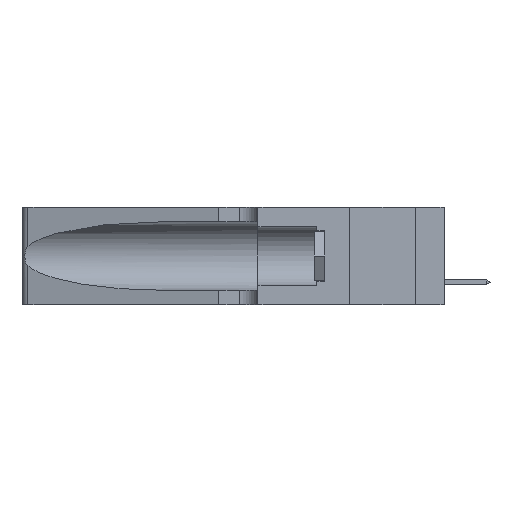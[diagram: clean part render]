
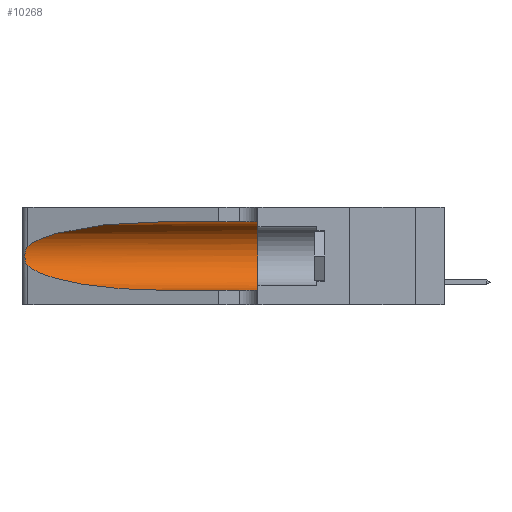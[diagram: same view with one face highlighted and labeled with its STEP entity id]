
A CAD part, left-side view. The second image highlights one B-rep face of the part: STEP entity #10268.
In plain terms, the highlighted cylindrical face has radius 3.308 mm (diameter 6.617 mm), a partial arc.
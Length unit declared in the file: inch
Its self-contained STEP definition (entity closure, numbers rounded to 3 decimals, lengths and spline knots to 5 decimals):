
#1275 = CARTESIAN_POINT ( 'NONE',  ( 0.1305, 0.72297, 0.05475 ) ) ;
#1622 = ORIENTED_EDGE ( 'NONE', *, *, #4920, .T. ) ;
#1725 = CARTESIAN_POINT ( 'NONE',  ( 0.26017, 1.23833, 0.17102 ) ) ;
#1914 = DIRECTION ( 'NONE',  ( 0., 0., -1. ) ) ;
#2087 = LINE ( 'NONE', #11786, #18415 ) ;
#2532 = CARTESIAN_POINT ( 'NONE',  ( 0.25787, 1.23484, 0.2124 ) ) ;
#2610 = CARTESIAN_POINT ( 'NONE',  ( 0.26075, 1.23896, 0.19203 ) ) ;
#3194 = CARTESIAN_POINT ( 'NONE',  ( 0.25487, 1.22718, 0.14631 ) ) ;
#3207 = ORIENTED_EDGE ( 'NONE', *, *, #10612, .T. ) ;
#3215 = CARTESIAN_POINT ( 'NONE',  ( 0.25487, 1.22718, 0.14631 ) ) ;
#3239 = CARTESIAN_POINT ( 'NONE',  ( 0.1305, 0.72297, 0.31525 ) ) ;
#3676 = CARTESIAN_POINT ( 'NONE',  ( 0.2373, 1.15595, 0.28018 ) ) ;
#4524 = EDGE_LOOP ( 'NONE', ( #3207, #1622, #17276, #13092, #5275, #13192 ) ) ;
#4920 = EDGE_CURVE ( 'NONE', #6369, #17514, #17441, .T. ) ;
#5008 = CARTESIAN_POINT ( 'NONE',  ( 0.1305, 1.61858, 0.185 ) ) ;
#5275 = ORIENTED_EDGE ( 'NONE', *, *, #12009, .F. ) ;
#5328 = DIRECTION ( 'NONE',  ( 0., -1., 0. ) ) ;
#5512 = VERTEX_POINT ( 'NONE', #19011 ) ;
#5813 = VERTEX_POINT ( 'NONE', #1275 ) ;
#5900 = FACE_OUTER_BOUND ( 'NONE', #4524, .T. ) ;
#5955 = EDGE_CURVE ( 'NONE', #17514, #5813, #17702, .T. ) ;
#6369 = VERTEX_POINT ( 'NONE', #16357 ) ;
#7639 = CYLINDRICAL_SURFACE ( 'NONE', #16530, 0.13025 ) ;
#7770 = EDGE_CURVE ( 'NONE', #17005, #5512, #19348, .T. ) ;
#9544 = CARTESIAN_POINT ( 'NONE',  ( 0.25856, 1.23593, 0.16098 ) ) ;
#9604 = CARTESIAN_POINT ( 'NONE',  ( 0.25789, 1.23486, 0.15765 ) ) ;
#9733 = CARTESIAN_POINT ( 'NONE',  ( 0.25487, 1.22718, 0.22369 ) ) ;
#9821 = CARTESIAN_POINT ( 'NONE',  ( 0.18966, 0.96281, 0.05475 ) ) ;
#9995 = VECTOR ( 'NONE', #5328, 39.37008 ) ;
#10268 = ADVANCED_FACE ( 'NONE', ( #5900 ), #7639, .F. ) ;
#10290 = CARTESIAN_POINT ( 'NONE',  ( 0.25487, 1.22718, 0.22369 ) ) ;
#10612 = EDGE_CURVE ( 'NONE', #17005, #6369, #12275, .T. ) ;
#11355 = CARTESIAN_POINT ( 'NONE',  ( 0.18966, 0.96281, 0.31525 ) ) ;
#11786 = CARTESIAN_POINT ( 'NONE',  ( 0.1305, 1.61858, 0.05475 ) ) ;
#12009 = EDGE_CURVE ( 'NONE', #5512, #19830, #14954, .T. ) ;
#12275 =( BOUNDED_CURVE ( )  B_SPLINE_CURVE ( 3, ( #19216, #11355, #3676, #9733 ),
 .UNSPECIFIED., .F., .F. ) 
 B_SPLINE_CURVE_WITH_KNOTS ( ( 4, 4 ),
 ( 1.5708, 2.84003 ),
 .UNSPECIFIED. ) 
 CURVE ( )  GEOMETRIC_REPRESENTATION_ITEM ( )  RATIONAL_B_SPLINE_CURVE ( ( 1., 0.87, 0.87, 1. ) ) 
 REPRESENTATION_ITEM ( '' )  );
#12307 = CARTESIAN_POINT ( 'NONE',  ( 0.2373, 1.15595, 0.08982 ) ) ;
#13092 = ORIENTED_EDGE ( 'NONE', *, *, #15916, .T. ) ;
#13192 = ORIENTED_EDGE ( 'NONE', *, *, #7770, .F. ) ;
#13518 = CARTESIAN_POINT ( 'NONE',  ( 0.1305, 0.35, 0.185 ) ) ;
#13603 = CARTESIAN_POINT ( 'NONE',  ( 0.25854, 1.2359, 0.20912 ) ) ;
#13604 = DIRECTION ( 'NONE',  ( 0., -1., 0. ) ) ;
#13668 = CARTESIAN_POINT ( 'NONE',  ( 0.25639, 1.23184, 0.21858 ) ) ;
#14804 = DIRECTION ( 'NONE',  ( 0., 0., 1. ) ) ;
#14954 = CIRCLE ( 'NONE', #19080, 0.13025 ) ;
#15630 = CARTESIAN_POINT ( 'NONE',  ( 0.1305, 0.35, 0.05475 ) ) ;
#15775 = CARTESIAN_POINT ( 'NONE',  ( 0.25639, 1.23186, 0.15144 ) ) ;
#15848 = CARTESIAN_POINT ( 'NONE',  ( 0.1305, 0.72297, 0.05475 ) ) ;
#15916 = EDGE_CURVE ( 'NONE', #5813, #19830, #2087, .T. ) ;
#16113 = DIRECTION ( 'NONE',  ( 0., -1., 0. ) ) ;
#16317 = DIRECTION ( 'NONE',  ( 0., 1., 0. ) ) ;
#16357 = CARTESIAN_POINT ( 'NONE',  ( 0.25487, 1.22718, 0.22369 ) ) ;
#16530 = AXIS2_PLACEMENT_3D ( 'NONE', #5008, #16113, #1914 ) ;
#17005 = VERTEX_POINT ( 'NONE', #3239 ) ;
#17276 = ORIENTED_EDGE ( 'NONE', *, *, #5955, .T. ) ;
#17441 = B_SPLINE_CURVE_WITH_KNOTS ( 'NONE', 3,
 ( #10290, #18287, #13668, #2532, #13603, #19928, #2610, #19030, #1725, #9544, #9604, #15775, #18973, #3215 ),
 .UNSPECIFIED., .F., .F.,
 ( 4, 2, 2, 2, 2, 2, 4 ),
 ( 0., 0.00027, 0.00053, 0.00107, 0.0016, 0.00187, 0.00214 ),
 .UNSPECIFIED. ) ;
#17514 = VERTEX_POINT ( 'NONE', #3194 ) ;
#17702 =( BOUNDED_CURVE ( )  B_SPLINE_CURVE ( 3, ( #20316, #12307, #9821, #15848 ),
 .UNSPECIFIED., .F., .T. ) 
 B_SPLINE_CURVE_WITH_KNOTS ( ( 4, 4 ),
 ( 3.44316, 4.71239 ),
 .UNSPECIFIED. ) 
 CURVE ( )  GEOMETRIC_REPRESENTATION_ITEM ( )  RATIONAL_B_SPLINE_CURVE ( ( 1., 0.87, 0.87, 1. ) ) 
 REPRESENTATION_ITEM ( '' )  );
#17909 = CARTESIAN_POINT ( 'NONE',  ( 0.1305, 1.61858, 0.31525 ) ) ;
#18287 = CARTESIAN_POINT ( 'NONE',  ( 0.25555, 1.22994, 0.2215 ) ) ;
#18415 = VECTOR ( 'NONE', #13604, 39.37008 ) ;
#18973 = CARTESIAN_POINT ( 'NONE',  ( 0.25555, 1.22993, 0.14849 ) ) ;
#19011 = CARTESIAN_POINT ( 'NONE',  ( 0.1305, 0.35, 0.31525 ) ) ;
#19030 = CARTESIAN_POINT ( 'NONE',  ( 0.26075, 1.23896, 0.178 ) ) ;
#19080 = AXIS2_PLACEMENT_3D ( 'NONE', #13518, #16317, #14804 ) ;
#19216 = CARTESIAN_POINT ( 'NONE',  ( 0.1305, 0.72297, 0.31525 ) ) ;
#19348 = LINE ( 'NONE', #17909, #9995 ) ;
#19830 = VERTEX_POINT ( 'NONE', #15630 ) ;
#19928 = CARTESIAN_POINT ( 'NONE',  ( 0.26018, 1.23835, 0.19895 ) ) ;
#20316 = CARTESIAN_POINT ( 'NONE',  ( 0.25487, 1.22718, 0.14631 ) ) ;
